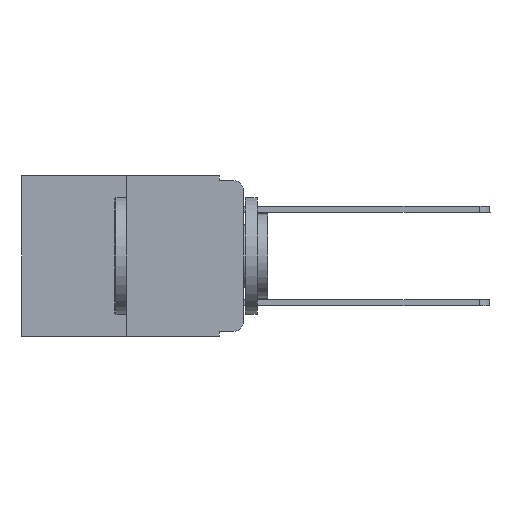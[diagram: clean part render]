
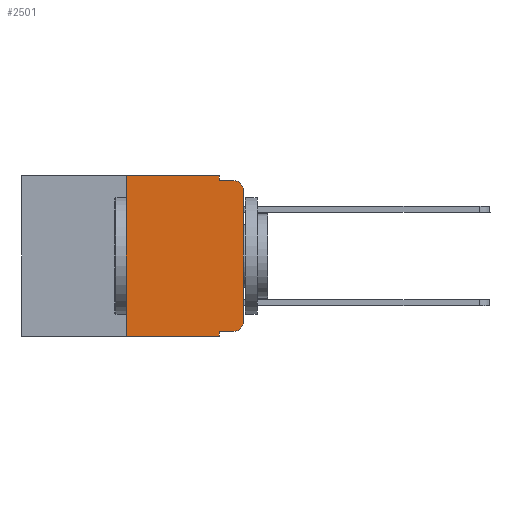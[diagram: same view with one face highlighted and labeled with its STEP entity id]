
A CAD part, left-side view. The second image highlights one B-rep face of the part: STEP entity #2501.
In plain terms, the highlighted planar face has unit normal (-1, 0, 0).
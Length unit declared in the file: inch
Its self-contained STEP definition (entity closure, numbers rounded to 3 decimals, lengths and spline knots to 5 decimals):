
#236 = AXIS2_PLACEMENT_3D ( 'NONE', #23583, #2780, #6432 ) ;
#499 = CARTESIAN_POINT ( 'NONE',  ( 0., 0.473, 0. ) ) ;
#1051 = EDGE_CURVE ( 'NONE', #22715, #1794, #17537, .T. ) ;
#1722 = EDGE_LOOP ( 'NONE', ( #7960, #23162, #8854, #6690, #4217, #3191, #20962, #16048, #14546, #7352 ) ) ;
#1794 = VERTEX_POINT ( 'NONE', #18578 ) ;
#2171 = VECTOR ( 'NONE', #9867, 39.37008 ) ;
#2467 = CARTESIAN_POINT ( 'NONE',  ( 0., 0.25, -0.343 ) ) ;
#2501 = ADVANCED_FACE ( 'NONE', ( #18046 ), #17944, .F. ) ;
#2651 = VECTOR ( 'NONE', #2732, 39.37008 ) ;
#2732 = DIRECTION ( 'NONE',  ( 0., -1., 0. ) ) ;
#2780 = DIRECTION ( 'NONE',  ( 1., 0., 0. ) ) ;
#3191 = ORIENTED_EDGE ( 'NONE', *, *, #3516, .F. ) ;
#3246 = CARTESIAN_POINT ( 'NONE',  ( 0., 0., -0.313 ) ) ;
#3516 = EDGE_CURVE ( 'NONE', #22300, #4972, #7271, .T. ) ;
#3976 = CARTESIAN_POINT ( 'NONE',  ( 0., 0.051, -0.333 ) ) ;
#4108 = VECTOR ( 'NONE', #5648, 39.37008 ) ;
#4217 = ORIENTED_EDGE ( 'NONE', *, *, #7048, .F. ) ;
#4666 = VECTOR ( 'NONE', #13915, 39.37008 ) ;
#4972 = VERTEX_POINT ( 'NONE', #16956 ) ;
#5648 = DIRECTION ( 'NONE',  ( 0., -1., 0. ) ) ;
#5923 = DIRECTION ( 'NONE',  ( 0., 0., -1. ) ) ;
#5930 = LINE ( 'NONE', #23372, #2651 ) ;
#6090 = EDGE_CURVE ( 'NONE', #22300, #1794, #5930, .T. ) ;
#6377 = EDGE_CURVE ( 'NONE', #19715, #12932, #8587, .T. ) ;
#6432 = DIRECTION ( 'NONE',  ( 0., 0., -1. ) ) ;
#6690 = ORIENTED_EDGE ( 'NONE', *, *, #13795, .F. ) ;
#7048 = EDGE_CURVE ( 'NONE', #4972, #12554, #18032, .T. ) ;
#7271 = LINE ( 'NONE', #13453, #2171 ) ;
#7315 = LINE ( 'NONE', #11717, #9082 ) ;
#7352 = ORIENTED_EDGE ( 'NONE', *, *, #18185, .T. ) ;
#7414 = VECTOR ( 'NONE', #22806, 39.37008 ) ;
#7643 = CARTESIAN_POINT ( 'NONE',  ( 0., 0., -0.03 ) ) ;
#7746 = DIRECTION ( 'NONE',  ( 0., 0., -1. ) ) ;
#7960 = ORIENTED_EDGE ( 'NONE', *, *, #8822, .T. ) ;
#8154 = DIRECTION ( 'NONE',  ( 0., -1., 0. ) ) ;
#8587 = LINE ( 'NONE', #17006, #4108 ) ;
#8822 = EDGE_CURVE ( 'NONE', #11265, #23314, #7315, .T. ) ;
#8854 = ORIENTED_EDGE ( 'NONE', *, *, #6377, .F. ) ;
#9082 = VECTOR ( 'NONE', #23798, 39.37008 ) ;
#9710 = DIRECTION ( 'NONE',  ( -1., 0., 0. ) ) ;
#9867 = DIRECTION ( 'NONE',  ( 0., 0., 1. ) ) ;
#10188 = CIRCLE ( 'NONE', #11487, 0.02 ) ;
#10989 = VERTEX_POINT ( 'NONE', #23632 ) ;
#11265 = VERTEX_POINT ( 'NONE', #3246 ) ;
#11487 = AXIS2_PLACEMENT_3D ( 'NONE', #17223, #17299, #11637 ) ;
#11637 = DIRECTION ( 'NONE',  ( 0., 0., -1. ) ) ;
#11717 = CARTESIAN_POINT ( 'NONE',  ( 0., 0., 0. ) ) ;
#12554 = VERTEX_POINT ( 'NONE', #22223 ) ;
#12932 = VERTEX_POINT ( 'NONE', #18217 ) ;
#13453 = CARTESIAN_POINT ( 'NONE',  ( 0., 0.25, 0. ) ) ;
#13795 = EDGE_CURVE ( 'NONE', #12554, #19715, #16561, .T. ) ;
#13915 = DIRECTION ( 'NONE',  ( 0., 0., -1. ) ) ;
#14546 = ORIENTED_EDGE ( 'NONE', *, *, #23703, .T. ) ;
#14580 = VECTOR ( 'NONE', #7746, 39.37008 ) ;
#16048 = ORIENTED_EDGE ( 'NONE', *, *, #1051, .F. ) ;
#16561 = LINE ( 'NONE', #21308, #4666 ) ;
#16956 = CARTESIAN_POINT ( 'NONE',  ( 0., 0.25, 0. ) ) ;
#17006 = CARTESIAN_POINT ( 'NONE',  ( 0., 0.051, -0.01 ) ) ;
#17223 = CARTESIAN_POINT ( 'NONE',  ( 0., 0.02, -0.03 ) ) ;
#17299 = DIRECTION ( 'NONE',  ( -1., 0., 0. ) ) ;
#17537 = LINE ( 'NONE', #19102, #14580 ) ;
#17944 = PLANE ( 'NONE',  #236 ) ;
#18032 = LINE ( 'NONE', #499, #22478 ) ;
#18046 = FACE_OUTER_BOUND ( 'NONE', #1722, .T. ) ;
#18185 = EDGE_CURVE ( 'NONE', #10989, #11265, #20976, .T. ) ;
#18217 = CARTESIAN_POINT ( 'NONE',  ( 0., 0.02, -0.01 ) ) ;
#18578 = CARTESIAN_POINT ( 'NONE',  ( 0., 0.051, -0.343 ) ) ;
#19101 = CARTESIAN_POINT ( 'NONE',  ( 0., 0.02, -0.313 ) ) ;
#19102 = CARTESIAN_POINT ( 'NONE',  ( 0., 0.051, 0. ) ) ;
#19599 = EDGE_CURVE ( 'NONE', #23314, #12932, #10188, .T. ) ;
#19715 = VERTEX_POINT ( 'NONE', #22916 ) ;
#20696 = AXIS2_PLACEMENT_3D ( 'NONE', #19101, #9710, #5923 ) ;
#20962 = ORIENTED_EDGE ( 'NONE', *, *, #6090, .T. ) ;
#20976 = CIRCLE ( 'NONE', #20696, 0.02 ) ;
#21308 = CARTESIAN_POINT ( 'NONE',  ( 0., 0.051, 0. ) ) ;
#21954 = LINE ( 'NONE', #3976, #7414 ) ;
#22223 = CARTESIAN_POINT ( 'NONE',  ( 0., 0.051, 0. ) ) ;
#22300 = VERTEX_POINT ( 'NONE', #2467 ) ;
#22453 = CARTESIAN_POINT ( 'NONE',  ( 0., 0.051, -0.333 ) ) ;
#22478 = VECTOR ( 'NONE', #8154, 39.37008 ) ;
#22715 = VERTEX_POINT ( 'NONE', #22453 ) ;
#22806 = DIRECTION ( 'NONE',  ( 0., -1., 0. ) ) ;
#22916 = CARTESIAN_POINT ( 'NONE',  ( 0., 0.051, -0.01 ) ) ;
#23162 = ORIENTED_EDGE ( 'NONE', *, *, #19599, .T. ) ;
#23314 = VERTEX_POINT ( 'NONE', #7643 ) ;
#23372 = CARTESIAN_POINT ( 'NONE',  ( 0., 0.473, -0.343 ) ) ;
#23583 = CARTESIAN_POINT ( 'NONE',  ( 0., 0.473, 0. ) ) ;
#23632 = CARTESIAN_POINT ( 'NONE',  ( 0., 0.02, -0.333 ) ) ;
#23703 = EDGE_CURVE ( 'NONE', #22715, #10989, #21954, .T. ) ;
#23798 = DIRECTION ( 'NONE',  ( 0., 0., 1. ) ) ;
